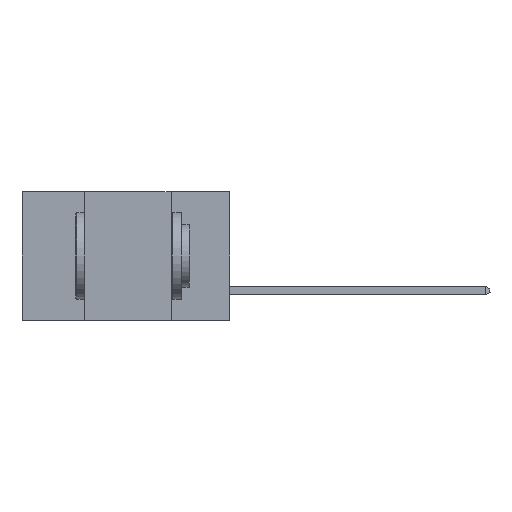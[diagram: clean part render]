
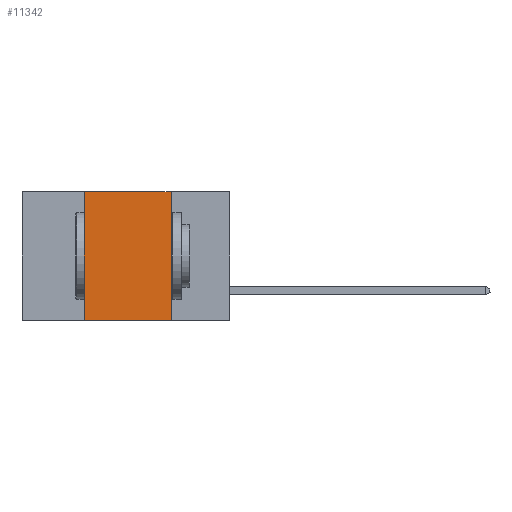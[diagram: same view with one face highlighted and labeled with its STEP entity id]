
A CAD part, left-side view. The second image highlights one B-rep face of the part: STEP entity #11342.
In plain terms, the highlighted planar face has unit normal (-1, 0, 0).
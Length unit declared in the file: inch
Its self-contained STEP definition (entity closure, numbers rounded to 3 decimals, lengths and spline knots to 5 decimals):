
#235 = VECTOR ( 'NONE', #3646, 39.37008 ) ;
#443 = CARTESIAN_POINT ( 'NONE',  ( 0., 0.17, 0. ) ) ;
#592 = FACE_OUTER_BOUND ( 'NONE', #11887, .T. ) ;
#781 = VERTEX_POINT ( 'NONE', #9357 ) ;
#1515 = CARTESIAN_POINT ( 'NONE',  ( 0., 0.17, -0.37 ) ) ;
#2302 = CARTESIAN_POINT ( 'NONE',  ( 0., 0.42, 0. ) ) ;
#2689 = VECTOR ( 'NONE', #9046, 39.37008 ) ;
#2842 = ORIENTED_EDGE ( 'NONE', *, *, #11896, .F. ) ;
#3017 = CARTESIAN_POINT ( 'NONE',  ( 0., 0.6, 0. ) ) ;
#3027 = EDGE_CURVE ( 'NONE', #781, #7048, #9441, .T. ) ;
#3478 = LINE ( 'NONE', #10191, #235 ) ;
#3646 = DIRECTION ( 'NONE',  ( 0., -1., 0. ) ) ;
#4156 = EDGE_CURVE ( 'NONE', #7369, #781, #11085, .T. ) ;
#4191 = DIRECTION ( 'NONE',  ( 0., -1., 0. ) ) ;
#4345 = ORIENTED_EDGE ( 'NONE', *, *, #3027, .F. ) ;
#4980 = VERTEX_POINT ( 'NONE', #1515 ) ;
#5720 = ORIENTED_EDGE ( 'NONE', *, *, #8976, .T. ) ;
#5965 = CARTESIAN_POINT ( 'NONE',  ( 0., 0.17, 0. ) ) ;
#6551 = LINE ( 'NONE', #443, #2689 ) ;
#7048 = VERTEX_POINT ( 'NONE', #5965 ) ;
#7369 = VERTEX_POINT ( 'NONE', #12050 ) ;
#7493 = VECTOR ( 'NONE', #11010, 39.37008 ) ;
#8232 = ORIENTED_EDGE ( 'NONE', *, *, #4156, .F. ) ;
#8697 = AXIS2_PLACEMENT_3D ( 'NONE', #3017, #9639, #10529 ) ;
#8976 = EDGE_CURVE ( 'NONE', #7369, #4980, #3478, .T. ) ;
#9046 = DIRECTION ( 'NONE',  ( 0., 0., -1. ) ) ;
#9357 = CARTESIAN_POINT ( 'NONE',  ( 0., 0.42, 0. ) ) ;
#9441 = LINE ( 'NONE', #9851, #11269 ) ;
#9639 = DIRECTION ( 'NONE',  ( 1., 0., 0. ) ) ;
#9851 = CARTESIAN_POINT ( 'NONE',  ( 0., 0.6, 0. ) ) ;
#10191 = CARTESIAN_POINT ( 'NONE',  ( 0., 0.6, -0.37 ) ) ;
#10529 = DIRECTION ( 'NONE',  ( 0., 0., -1. ) ) ;
#10611 = PLANE ( 'NONE',  #8697 ) ;
#11010 = DIRECTION ( 'NONE',  ( 0., 0., 1. ) ) ;
#11085 = LINE ( 'NONE', #2302, #7493 ) ;
#11269 = VECTOR ( 'NONE', #4191, 39.37008 ) ;
#11342 = ADVANCED_FACE ( 'NONE', ( #592 ), #10611, .F. ) ;
#11887 = EDGE_LOOP ( 'NONE', ( #2842, #4345, #8232, #5720 ) ) ;
#11896 = EDGE_CURVE ( 'NONE', #7048, #4980, #6551, .T. ) ;
#12050 = CARTESIAN_POINT ( 'NONE',  ( 0., 0.42, -0.37 ) ) ;
